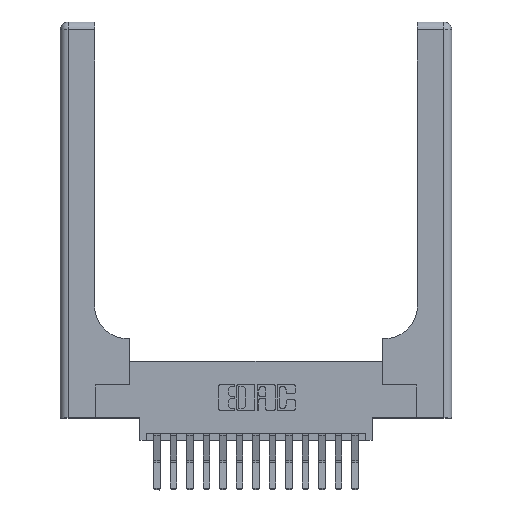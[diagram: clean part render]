
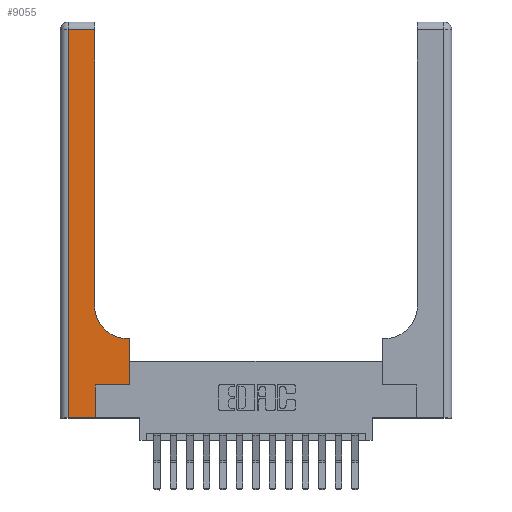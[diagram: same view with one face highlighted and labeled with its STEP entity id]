
A CAD part, top view. The second image highlights one B-rep face of the part: STEP entity #9055.
In plain terms, the highlighted planar face has unit normal (0, 0, 1).
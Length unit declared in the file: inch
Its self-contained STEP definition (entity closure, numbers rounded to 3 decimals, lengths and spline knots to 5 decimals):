
#238 = CARTESIAN_POINT ( 'NONE',  ( 0.26, 2.94, 0.37 ) ) ;
#493 = VERTEX_POINT ( 'NONE', #238 ) ;
#1281 = CARTESIAN_POINT ( 'NONE',  ( 0., 2.94, 0.37 ) ) ;
#1324 = LINE ( 'NONE', #11151, #12298 ) ;
#1393 = DIRECTION ( 'NONE',  ( 0., 1., 0. ) ) ;
#1546 = VERTEX_POINT ( 'NONE', #8046 ) ;
#1867 = DIRECTION ( 'NONE',  ( 0., 0., -1. ) ) ;
#2126 = ORIENTED_EDGE ( 'NONE', *, *, #4202, .T. ) ;
#2317 = DIRECTION ( 'NONE',  ( 0., 1., 0. ) ) ;
#2467 = ORIENTED_EDGE ( 'NONE', *, *, #11244, .T. ) ;
#2517 = EDGE_CURVE ( 'NONE', #14397, #16611, #17109, .T. ) ;
#2580 = LINE ( 'NONE', #11614, #17573 ) ;
#2687 = DIRECTION ( 'NONE',  ( -1., 0., 0. ) ) ;
#3179 = AXIS2_PLACEMENT_3D ( 'NONE', #10087, #1867, #11488 ) ;
#3252 = EDGE_CURVE ( 'NONE', #15579, #1546, #6891, .T. ) ;
#3318 = VECTOR ( 'NONE', #12009, 39.37008 ) ;
#3346 = ORIENTED_EDGE ( 'NONE', *, *, #4010, .T. ) ;
#3398 = DIRECTION ( 'NONE',  ( 1., 0., 0. ) ) ;
#3730 = EDGE_CURVE ( 'NONE', #4686, #10821, #16391, .T. ) ;
#4010 = EDGE_CURVE ( 'NONE', #16611, #493, #6233, .T. ) ;
#4151 = EDGE_LOOP ( 'NONE', ( #3346, #5333, #13049, #4728, #2126, #11823, #5791, #2467, #5872 ) ) ;
#4202 = EDGE_CURVE ( 'NONE', #10821, #14471, #17730, .T. ) ;
#4293 = LINE ( 'NONE', #1281, #14756 ) ;
#4686 = VERTEX_POINT ( 'NONE', #10512 ) ;
#4728 = ORIENTED_EDGE ( 'NONE', *, *, #3730, .T. ) ;
#4951 = CARTESIAN_POINT ( 'NONE',  ( 0.265, 0., 0.37 ) ) ;
#5333 = ORIENTED_EDGE ( 'NONE', *, *, #14948, .T. ) ;
#5791 = ORIENTED_EDGE ( 'NONE', *, *, #3252, .T. ) ;
#5841 = CARTESIAN_POINT ( 'NONE',  ( 0.26, 0.85, 0.37 ) ) ;
#5872 = ORIENTED_EDGE ( 'NONE', *, *, #2517, .T. ) ;
#6233 = LINE ( 'NONE', #6555, #7077 ) ;
#6364 = CARTESIAN_POINT ( 'NONE',  ( 0.51, 0.6, 0.37 ) ) ;
#6555 = CARTESIAN_POINT ( 'NONE',  ( 0.26, 3., 0.37 ) ) ;
#6888 = EDGE_CURVE ( 'NONE', #13647, #4686, #6981, .T. ) ;
#6891 = LINE ( 'NONE', #15912, #14171 ) ;
#6898 = CARTESIAN_POINT ( 'NONE',  ( 0.265, 0., 0.37 ) ) ;
#6981 = LINE ( 'NONE', #7889, #3318 ) ;
#7077 = VECTOR ( 'NONE', #2317, 39.37008 ) ;
#7098 = DIRECTION ( 'NONE',  ( 0., 0., -1. ) ) ;
#7367 = CARTESIAN_POINT ( 'NONE',  ( 0.528, 0.25, 0.37 ) ) ;
#7889 = CARTESIAN_POINT ( 'NONE',  ( 0.06, 3., 0.37 ) ) ;
#8046 = CARTESIAN_POINT ( 'NONE',  ( 0.528, 0.6, 0.37 ) ) ;
#8627 = EDGE_CURVE ( 'NONE', #14471, #15579, #2580, .T. ) ;
#9055 = ADVANCED_FACE ( 'NONE', ( #11181 ), #9781, .F. ) ;
#9781 = PLANE ( 'NONE',  #14162 ) ;
#10087 = CARTESIAN_POINT ( 'NONE',  ( 0.51, 0.85, 0.37 ) ) ;
#10512 = CARTESIAN_POINT ( 'NONE',  ( 0.06, 0., 0.37 ) ) ;
#10821 = VERTEX_POINT ( 'NONE', #4951 ) ;
#11151 = CARTESIAN_POINT ( 'NONE',  ( 0.26, 0.6, 0.37 ) ) ;
#11181 = FACE_OUTER_BOUND ( 'NONE', #4151, .T. ) ;
#11244 = EDGE_CURVE ( 'NONE', #1546, #14397, #1324, .T. ) ;
#11488 = DIRECTION ( 'NONE',  ( 1., 0., 0. ) ) ;
#11614 = CARTESIAN_POINT ( 'NONE',  ( 0.265, 0.25, 0.37 ) ) ;
#11823 = ORIENTED_EDGE ( 'NONE', *, *, #8627, .T. ) ;
#11962 = CARTESIAN_POINT ( 'NONE',  ( 0.265, 0.25, 0.37 ) ) ;
#11988 = CARTESIAN_POINT ( 'NONE',  ( 0., 0., 0.37 ) ) ;
#12009 = DIRECTION ( 'NONE',  ( 0., -1., 0. ) ) ;
#12298 = VECTOR ( 'NONE', #12527, 39.37008 ) ;
#12527 = DIRECTION ( 'NONE',  ( -1., 0., 0. ) ) ;
#12786 = VECTOR ( 'NONE', #14730, 39.37008 ) ;
#13049 = ORIENTED_EDGE ( 'NONE', *, *, #6888, .T. ) ;
#13647 = VERTEX_POINT ( 'NONE', #15907 ) ;
#14162 = AXIS2_PLACEMENT_3D ( 'NONE', #15286, #7098, #16648 ) ;
#14171 = VECTOR ( 'NONE', #17274, 39.37008 ) ;
#14397 = VERTEX_POINT ( 'NONE', #6364 ) ;
#14471 = VERTEX_POINT ( 'NONE', #11962 ) ;
#14557 = VECTOR ( 'NONE', #1393, 39.37008 ) ;
#14730 = DIRECTION ( 'NONE',  ( 1., 0., 0. ) ) ;
#14756 = VECTOR ( 'NONE', #2687, 39.37008 ) ;
#14948 = EDGE_CURVE ( 'NONE', #493, #13647, #4293, .T. ) ;
#15286 = CARTESIAN_POINT ( 'NONE',  ( 0., 3., 0.37 ) ) ;
#15579 = VERTEX_POINT ( 'NONE', #7367 ) ;
#15907 = CARTESIAN_POINT ( 'NONE',  ( 0.06, 2.94, 0.37 ) ) ;
#15912 = CARTESIAN_POINT ( 'NONE',  ( 0.528, 0.25, 0.37 ) ) ;
#16391 = LINE ( 'NONE', #11988, #12786 ) ;
#16611 = VERTEX_POINT ( 'NONE', #5841 ) ;
#16648 = DIRECTION ( 'NONE',  ( -1., 0., 0. ) ) ;
#17109 = CIRCLE ( 'NONE', #3179, 0.25 ) ;
#17274 = DIRECTION ( 'NONE',  ( 0., 1., 0. ) ) ;
#17573 = VECTOR ( 'NONE', #3398, 39.37008 ) ;
#17730 = LINE ( 'NONE', #6898, #14557 ) ;
